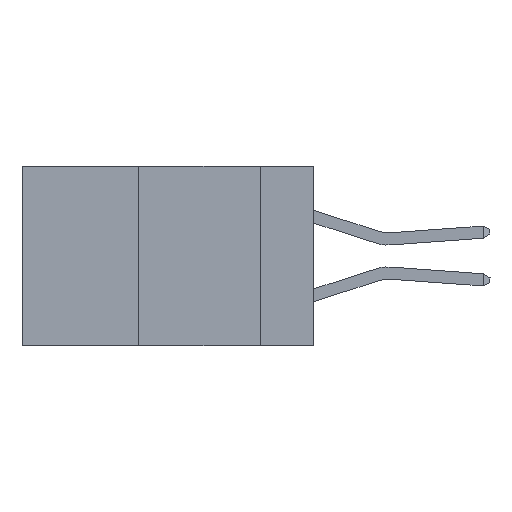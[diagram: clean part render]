
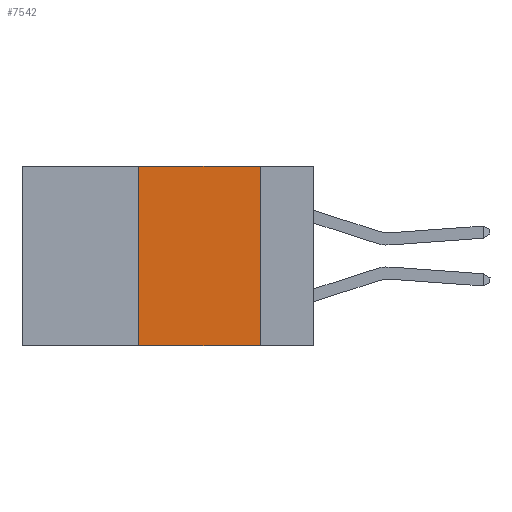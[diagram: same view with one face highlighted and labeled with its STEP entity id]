
A CAD part, left-side view. The second image highlights one B-rep face of the part: STEP entity #7542.
In plain terms, the highlighted planar face has unit normal (-1, 0, 0).
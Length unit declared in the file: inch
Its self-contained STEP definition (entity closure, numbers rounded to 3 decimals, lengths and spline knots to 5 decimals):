
#378 = VECTOR ( 'NONE', #15291, 39.37008 ) ;
#972 = AXIS2_PLACEMENT_3D ( 'NONE', #10049, #1856, #11394 ) ;
#989 = VERTEX_POINT ( 'NONE', #5074 ) ;
#1856 = DIRECTION ( 'NONE',  ( 1., 0., 0. ) ) ;
#2353 = EDGE_CURVE ( 'NONE', #15769, #6690, #15709, .T. ) ;
#3763 = DIRECTION ( 'NONE',  ( 0., 0., -1. ) ) ;
#3859 = EDGE_CURVE ( 'NONE', #14284, #6690, #12897, .T. ) ;
#4230 = CARTESIAN_POINT ( 'NONE',  ( 0., 0.11, -0.37 ) ) ;
#4495 = LINE ( 'NONE', #4597, #378 ) ;
#4597 = CARTESIAN_POINT ( 'NONE',  ( 0., 0.36, 0. ) ) ;
#5074 = CARTESIAN_POINT ( 'NONE',  ( 0., 0.36, 0. ) ) ;
#5423 = CARTESIAN_POINT ( 'NONE',  ( 0., 0.11, 0. ) ) ;
#6690 = VERTEX_POINT ( 'NONE', #4230 ) ;
#6781 = CARTESIAN_POINT ( 'NONE',  ( 0., 0.6, 0. ) ) ;
#7302 = DIRECTION ( 'NONE',  ( 0., -1., 0. ) ) ;
#7542 = ADVANCED_FACE ( 'NONE', ( #14996 ), #12640, .F. ) ;
#7889 = LINE ( 'NONE', #6781, #14529 ) ;
#8486 = VECTOR ( 'NONE', #7302, 39.37008 ) ;
#8648 = VECTOR ( 'NONE', #3763, 39.37008 ) ;
#8749 = EDGE_CURVE ( 'NONE', #14284, #989, #4495, .T. ) ;
#9481 = DIRECTION ( 'NONE',  ( 0., -1., 0. ) ) ;
#10049 = CARTESIAN_POINT ( 'NONE',  ( 0., 0.6, 0. ) ) ;
#10804 = EDGE_LOOP ( 'NONE', ( #17118, #17208, #17236, #17344 ) ) ;
#11394 = DIRECTION ( 'NONE',  ( 0., 0., -1. ) ) ;
#11882 = CARTESIAN_POINT ( 'NONE',  ( 0., 0.11, 0. ) ) ;
#12640 = PLANE ( 'NONE',  #972 ) ;
#12897 = LINE ( 'NONE', #13933, #8486 ) ;
#13933 = CARTESIAN_POINT ( 'NONE',  ( 0., 0.6, -0.37 ) ) ;
#14284 = VERTEX_POINT ( 'NONE', #14706 ) ;
#14529 = VECTOR ( 'NONE', #9481, 39.37008 ) ;
#14706 = CARTESIAN_POINT ( 'NONE',  ( 0., 0.36, -0.37 ) ) ;
#14996 = FACE_OUTER_BOUND ( 'NONE', #10804, .T. ) ;
#15291 = DIRECTION ( 'NONE',  ( 0., 0., 1. ) ) ;
#15709 = LINE ( 'NONE', #11882, #8648 ) ;
#15769 = VERTEX_POINT ( 'NONE', #5423 ) ;
#15776 = EDGE_CURVE ( 'NONE', #989, #15769, #7889, .T. ) ;
#17118 = ORIENTED_EDGE ( 'NONE', *, *, #2353, .F. ) ;
#17208 = ORIENTED_EDGE ( 'NONE', *, *, #15776, .F. ) ;
#17236 = ORIENTED_EDGE ( 'NONE', *, *, #8749, .F. ) ;
#17344 = ORIENTED_EDGE ( 'NONE', *, *, #3859, .T. ) ;
